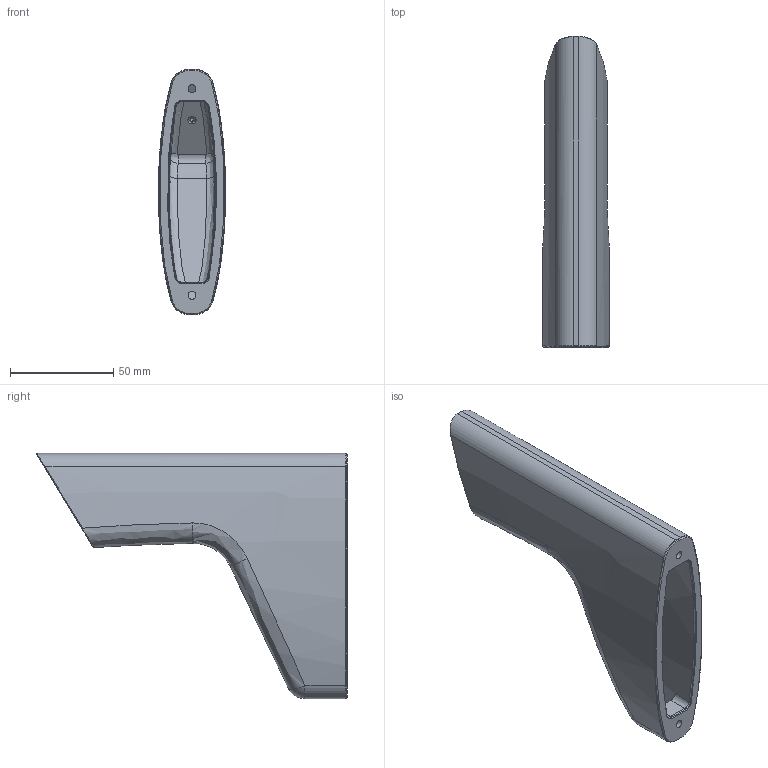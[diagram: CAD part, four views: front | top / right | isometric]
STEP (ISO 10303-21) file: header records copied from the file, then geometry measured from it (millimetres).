
FILE_DESCRIPTION(/* description */ (''),/* implementation_level */ '2;1');
FILE_NAME(/* name */ 'Stock Half 1.step',/* time_stamp */ '2021-10-03T07:00:13-04:00',/* author */ (''),/* organization */ (''),/* preprocessor_version */ 'ST-DEVELOPER v18.1',/* originating_system */ 'Autodesk Translation Framework v10.10.0.1391',/* authorisation */ '');
FILE_SCHEMA (('AUTOMOTIVE_DESIGN { 1 0 10303 214 3 1 1 }'));
Length unit declared in the file: millimetre
Products named in the file (1): Stock Half 1
Bounding box: 32.39 x 150.34 x 118.61 mm (x, y, z)
Volume: 125370.2 mm3; surface area: 46857.5 mm2
Topology: 1 solids, 1 shells, 196 faces, 429 edges, 247 vertices
Faces by surface type: bspline 119, cylinder 35, plane 26, sphere 8, cone 4, torus 4
Full cylindrical faces by diameter (mm): 1.952 x1, 2 x1, 3.8 x2, 6.7 x4
Entity records: 9490 total; most frequent: CARTESIAN_POINT 5820, ORIENTED_EDGE 858, DIRECTION 526, EDGE_CURVE 429, VERTEX_POINT 247, EDGE_LOOP 214, AXIS2_PLACEMENT_3D 207, FACE_OUTER_BOUND 196
